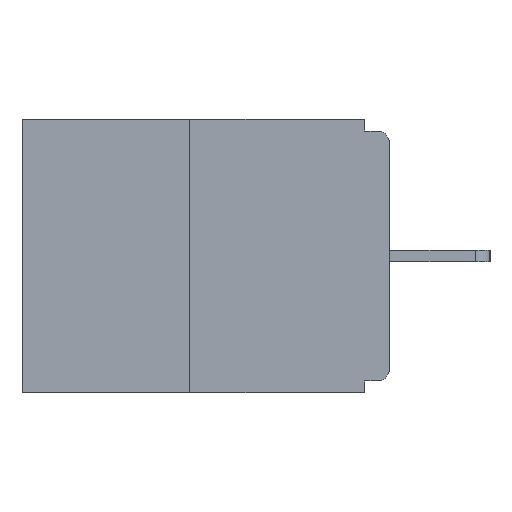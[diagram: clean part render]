
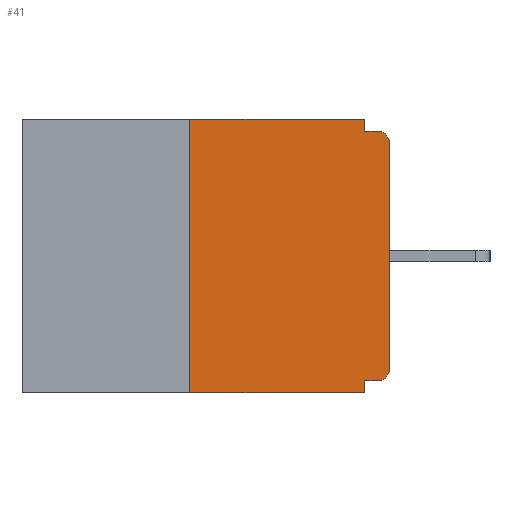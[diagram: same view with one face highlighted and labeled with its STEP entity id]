
A CAD part, left-side view. The second image highlights one B-rep face of the part: STEP entity #41.
In plain terms, the highlighted planar face has unit normal (-1, 0, 0).
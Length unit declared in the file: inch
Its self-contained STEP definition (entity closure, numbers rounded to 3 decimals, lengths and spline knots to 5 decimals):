
#41 = ADVANCED_FACE ( 'NONE', ( #10877 ), #6340, .F. ) ;
#43 = CARTESIAN_POINT ( 'NONE',  ( 0., 0.25, 0. ) ) ;
#405 = LINE ( 'NONE', #1485, #2988 ) ;
#428 = CARTESIAN_POINT ( 'NONE',  ( 0., 0., -0.328 ) ) ;
#548 = EDGE_CURVE ( 'NONE', #3836, #990, #9025, .T. ) ;
#990 = VERTEX_POINT ( 'NONE', #4673 ) ;
#1088 = VERTEX_POINT ( 'NONE', #8681 ) ;
#1168 = VERTEX_POINT ( 'NONE', #6112 ) ;
#1485 = CARTESIAN_POINT ( 'NONE',  ( 0., 0.031, 0. ) ) ;
#1495 = ORIENTED_EDGE ( 'NONE', *, *, #7877, .F. ) ;
#1629 = CIRCLE ( 'NONE', #8330, 0.015 ) ;
#1827 = LINE ( 'NONE', #11099, #2239 ) ;
#1916 = LINE ( 'NONE', #8270, #10321 ) ;
#1968 = EDGE_CURVE ( 'NONE', #11691, #1168, #5054, .T. ) ;
#2177 = EDGE_CURVE ( 'NONE', #10646, #3559, #1916, .T. ) ;
#2239 = VECTOR ( 'NONE', #2905, 39.37008 ) ;
#2288 = EDGE_CURVE ( 'NONE', #1168, #11046, #11477, .T. ) ;
#2671 = LINE ( 'NONE', #5255, #3938 ) ;
#2796 = DIRECTION ( 'NONE',  ( 0., 0., -1. ) ) ;
#2844 = LINE ( 'NONE', #6554, #10846 ) ;
#2892 = DIRECTION ( 'NONE',  ( 0., 0., -1. ) ) ;
#2905 = DIRECTION ( 'NONE',  ( 0., -1., 0. ) ) ;
#2988 = VECTOR ( 'NONE', #5873, 39.37008 ) ;
#3295 = CARTESIAN_POINT ( 'NONE',  ( 0., 0.031, -0.343 ) ) ;
#3307 = DIRECTION ( 'NONE',  ( 0., 0., -1. ) ) ;
#3559 = VERTEX_POINT ( 'NONE', #43 ) ;
#3615 = EDGE_CURVE ( 'NONE', #1088, #990, #10338, .T. ) ;
#3793 = CARTESIAN_POINT ( 'NONE',  ( 0., 0.015, -0.313 ) ) ;
#3796 = ORIENTED_EDGE ( 'NONE', *, *, #548, .T. ) ;
#3836 = VERTEX_POINT ( 'NONE', #5369 ) ;
#3853 = EDGE_CURVE ( 'NONE', #3559, #4431, #2844, .T. ) ;
#3901 = ORIENTED_EDGE ( 'NONE', *, *, #8548, .T. ) ;
#3911 = VECTOR ( 'NONE', #9381, 39.37008 ) ;
#3938 = VECTOR ( 'NONE', #7171, 39.37008 ) ;
#4431 = VERTEX_POINT ( 'NONE', #4738 ) ;
#4673 = CARTESIAN_POINT ( 'NONE',  ( 0., 0.015, -0.015 ) ) ;
#4738 = CARTESIAN_POINT ( 'NONE',  ( 0., 0.031, 0. ) ) ;
#4990 = DIRECTION ( 'NONE',  ( -1., 0., 0. ) ) ;
#5054 = LINE ( 'NONE', #428, #8023 ) ;
#5255 = CARTESIAN_POINT ( 'NONE',  ( 0., 0., 0. ) ) ;
#5270 = CARTESIAN_POINT ( 'NONE',  ( 0., 0.031, -0.343 ) ) ;
#5369 = CARTESIAN_POINT ( 'NONE',  ( 0., 0., -0.03 ) ) ;
#5636 = DIRECTION ( 'NONE',  ( 0., 0., 1. ) ) ;
#5678 = CARTESIAN_POINT ( 'NONE',  ( 0., 0., -0.015 ) ) ;
#5873 = DIRECTION ( 'NONE',  ( 0., 0., -1. ) ) ;
#5937 = ORIENTED_EDGE ( 'NONE', *, *, #2177, .F. ) ;
#5943 = CARTESIAN_POINT ( 'NONE',  ( 0., 0., -0.313 ) ) ;
#6009 = CARTESIAN_POINT ( 'NONE',  ( 0., 0.015, -0.03 ) ) ;
#6112 = CARTESIAN_POINT ( 'NONE',  ( 0., 0.031, -0.328 ) ) ;
#6340 = PLANE ( 'NONE',  #10909 ) ;
#6447 = DIRECTION ( 'NONE',  ( 0., -1., 0. ) ) ;
#6554 = CARTESIAN_POINT ( 'NONE',  ( 0., 0.46, 0. ) ) ;
#6723 = ORIENTED_EDGE ( 'NONE', *, *, #8375, .T. ) ;
#6967 = DIRECTION ( 'NONE',  ( 0., 1., 0. ) ) ;
#7047 = ORIENTED_EDGE ( 'NONE', *, *, #7402, .T. ) ;
#7171 = DIRECTION ( 'NONE',  ( 0., 0., 1. ) ) ;
#7211 = CARTESIAN_POINT ( 'NONE',  ( 0., 0.25, -0.343 ) ) ;
#7402 = EDGE_CURVE ( 'NONE', #11691, #7419, #1629, .T. ) ;
#7419 = VERTEX_POINT ( 'NONE', #5943 ) ;
#7521 = ORIENTED_EDGE ( 'NONE', *, *, #1968, .F. ) ;
#7877 = EDGE_CURVE ( 'NONE', #4431, #1088, #405, .T. ) ;
#8023 = VECTOR ( 'NONE', #6967, 39.37008 ) ;
#8270 = CARTESIAN_POINT ( 'NONE',  ( 0., 0.25, 0. ) ) ;
#8330 = AXIS2_PLACEMENT_3D ( 'NONE', #3793, #10307, #2892 ) ;
#8375 = EDGE_CURVE ( 'NONE', #7419, #3836, #2671, .T. ) ;
#8460 = AXIS2_PLACEMENT_3D ( 'NONE', #6009, #4990, #3307 ) ;
#8548 = EDGE_CURVE ( 'NONE', #10646, #11046, #1827, .T. ) ;
#8664 = EDGE_LOOP ( 'NONE', ( #10491, #5937, #3901, #8733, #7521, #7047, #6723, #3796, #9452, #1495 ) ) ;
#8681 = CARTESIAN_POINT ( 'NONE',  ( 0., 0.031, -0.015 ) ) ;
#8733 = ORIENTED_EDGE ( 'NONE', *, *, #2288, .F. ) ;
#9025 = CIRCLE ( 'NONE', #8460, 0.015 ) ;
#9381 = DIRECTION ( 'NONE',  ( 0., -1., 0. ) ) ;
#9452 = ORIENTED_EDGE ( 'NONE', *, *, #3615, .F. ) ;
#9633 = DIRECTION ( 'NONE',  ( 0., 0., -1. ) ) ;
#9913 = DIRECTION ( 'NONE',  ( 1., 0., 0. ) ) ;
#10307 = DIRECTION ( 'NONE',  ( -1., 0., 0. ) ) ;
#10321 = VECTOR ( 'NONE', #5636, 39.37008 ) ;
#10338 = LINE ( 'NONE', #5678, #3911 ) ;
#10491 = ORIENTED_EDGE ( 'NONE', *, *, #3853, .F. ) ;
#10646 = VERTEX_POINT ( 'NONE', #7211 ) ;
#10717 = VECTOR ( 'NONE', #9633, 39.37008 ) ;
#10819 = CARTESIAN_POINT ( 'NONE',  ( 0., 0.46, 0. ) ) ;
#10846 = VECTOR ( 'NONE', #6447, 39.37008 ) ;
#10877 = FACE_OUTER_BOUND ( 'NONE', #8664, .T. ) ;
#10909 = AXIS2_PLACEMENT_3D ( 'NONE', #10819, #9913, #2796 ) ;
#11046 = VERTEX_POINT ( 'NONE', #5270 ) ;
#11099 = CARTESIAN_POINT ( 'NONE',  ( 0., 0.46, -0.343 ) ) ;
#11477 = LINE ( 'NONE', #3295, #10717 ) ;
#11691 = VERTEX_POINT ( 'NONE', #11756 ) ;
#11756 = CARTESIAN_POINT ( 'NONE',  ( 0., 0.015, -0.328 ) ) ;
